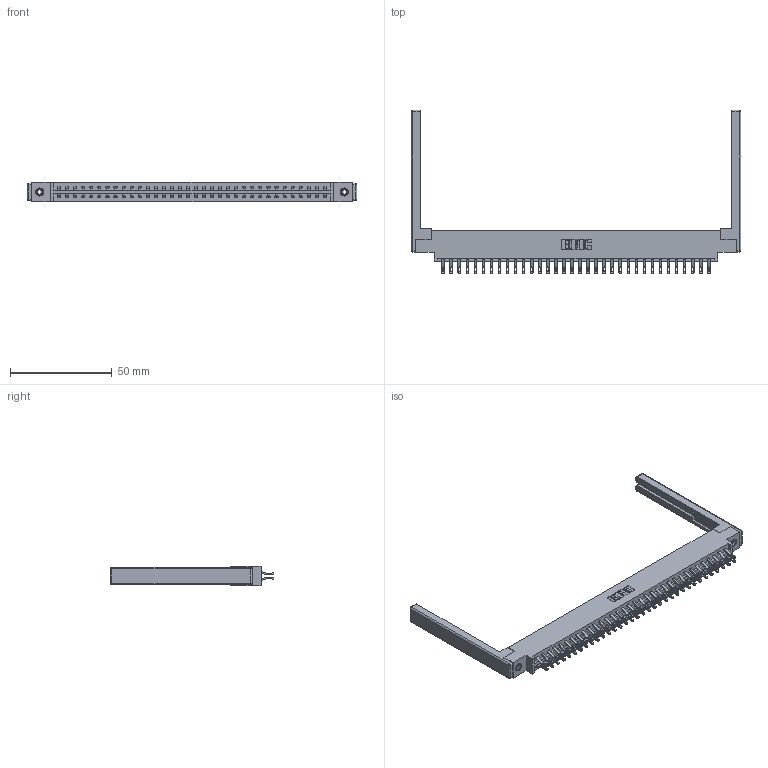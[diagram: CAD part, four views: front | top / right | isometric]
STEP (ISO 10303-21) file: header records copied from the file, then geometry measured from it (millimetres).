
FILE_DESCRIPTION (( 'STEP AP203' ), '1' );
FILE_NAME ('387-068-555-868.STEP', '2019-10-19T21:42:34', ( '' ), ( '' ), 'SwSTEP 2.0', 'SolidWorks 2016', '' );
FILE_SCHEMA (( 'CONFIG_CONTROL_DESIGN' ));
Length unit declared in the file: inch
Products named in the file (5): 345-292-001_555 Tail; 345-250-001_345-250-001-102; 387-068-555-868; 337 Part_0.170 Offset - 0.156 Dia-TI; 307-220-068
Assembly tree (73 placements, depth 2):
  387-068-555-868
    337 Part_0.170 Offset - 0.156 Dia-TI
    345-292-001_555 Tail  x68
    345-250-001_345-250-001-102  x2
    307-220-068  x2
Bounding box: 162.15 x 80.52 x 9.4 mm (x, y, z)
Volume: 21447.1 mm3; surface area: 24096.7 mm2
Topology: 73 solids, 73 shells, 4352 faces, 13565 edges, 9022 vertices
Faces by surface type: plane 2610, cylinder 1718, cone 12, sphere 8, torus 4
Entity records: 30614 total; most frequent: CARTESIAN_POINT 5165, ORIENTED_EDGE 5060, DIRECTION 4448, EDGE_CURVE 2530, VECTOR 2332, LINE 2332, VERTEX_POINT 1678, AXIS2_PLACEMENT_3D 1058
